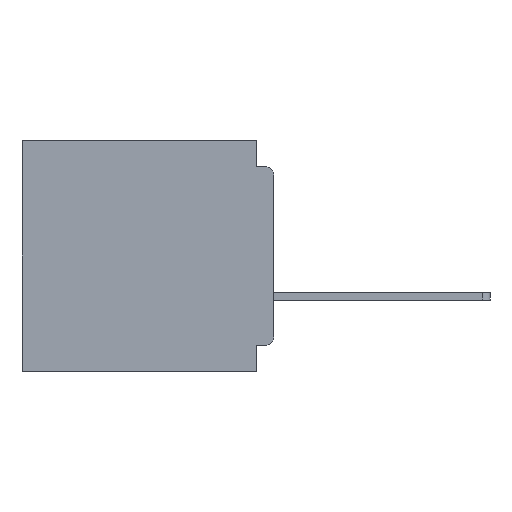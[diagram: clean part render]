
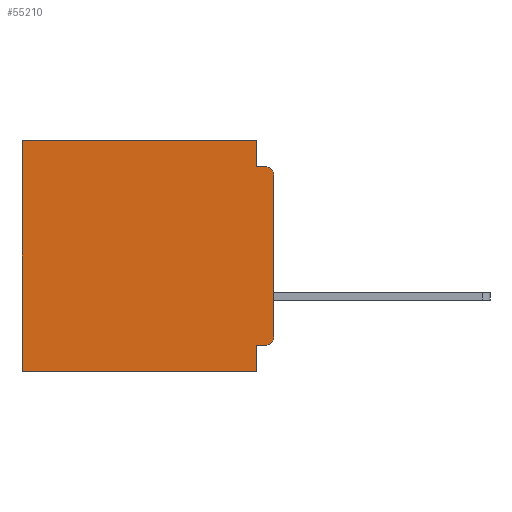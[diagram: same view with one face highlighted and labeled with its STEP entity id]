
A CAD part, left-side view. The second image highlights one B-rep face of the part: STEP entity #55210.
In plain terms, the highlighted planar face has unit normal (-1, 0, 0).
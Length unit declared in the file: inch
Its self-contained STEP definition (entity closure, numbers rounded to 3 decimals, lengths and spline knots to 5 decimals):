
#188 = VERTEX_POINT ( 'NONE', #54614 ) ;
#977 = VECTOR ( 'NONE', #39363, 39.37008 ) ;
#2365 = DIRECTION ( 'NONE',  ( -1., 0., 0. ) ) ;
#2395 = ORIENTED_EDGE ( 'NONE', *, *, #59650, .F. ) ;
#2439 = VERTEX_POINT ( 'NONE', #23832 ) ;
#3123 = CARTESIAN_POINT ( 'NONE',  ( 0.3, 0.031, -0.4 ) ) ;
#3156 = ORIENTED_EDGE ( 'NONE', *, *, #58411, .T. ) ;
#3273 = ORIENTED_EDGE ( 'NONE', *, *, #16764, .T. ) ;
#4020 = ORIENTED_EDGE ( 'NONE', *, *, #51384, .F. ) ;
#4127 = LINE ( 'NONE', #34115, #977 ) ;
#4299 = VERTEX_POINT ( 'NONE', #32899 ) ;
#4780 = DIRECTION ( 'NONE',  ( 0., -1., 0. ) ) ;
#5477 = LINE ( 'NONE', #53303, #43898 ) ;
#5922 = EDGE_LOOP ( 'NONE', ( #36828, #3156, #2395, #48694, #37758, #15868, #4020, #22206, #10386, #3273 ) ) ;
#6091 = VERTEX_POINT ( 'NONE', #54589 ) ;
#6470 = EDGE_CURVE ( 'NONE', #27082, #53759, #19765, .T. ) ;
#8656 = VERTEX_POINT ( 'NONE', #11162 ) ;
#10386 = ORIENTED_EDGE ( 'NONE', *, *, #46397, .F. ) ;
#10710 = DIRECTION ( 'NONE',  ( 0., 1., 0. ) ) ;
#11162 = CARTESIAN_POINT ( 'NONE',  ( 0.3, 0.015, -0.045 ) ) ;
#11356 = DIRECTION ( 'NONE',  ( -1., 0., 0. ) ) ;
#14209 = VERTEX_POINT ( 'NONE', #3123 ) ;
#14548 = CARTESIAN_POINT ( 'NONE',  ( 0.3, 0.031, -0.4 ) ) ;
#15117 = VERTEX_POINT ( 'NONE', #15348 ) ;
#15348 = CARTESIAN_POINT ( 'NONE',  ( 0.3, 0., -0.34 ) ) ;
#15868 = ORIENTED_EDGE ( 'NONE', *, *, #6470, .T. ) ;
#16097 = DIRECTION ( 'NONE',  ( 0., 1., 0. ) ) ;
#16764 = EDGE_CURVE ( 'NONE', #188, #15117, #54181, .T. ) ;
#18435 = DIRECTION ( 'NONE',  ( 1., 0., 0. ) ) ;
#19655 = DIRECTION ( 'NONE',  ( 0., 0., -1. ) ) ;
#19765 = LINE ( 'NONE', #42918, #31471 ) ;
#20411 = EDGE_CURVE ( 'NONE', #2439, #15117, #5477, .T. ) ;
#22071 = VECTOR ( 'NONE', #28201, 39.37008 ) ;
#22206 = ORIENTED_EDGE ( 'NONE', *, *, #30041, .F. ) ;
#23205 = CARTESIAN_POINT ( 'NONE',  ( 0.3, 0., -0.355 ) ) ;
#23832 = CARTESIAN_POINT ( 'NONE',  ( 0.3, 0., -0.06 ) ) ;
#24019 = EDGE_CURVE ( 'NONE', #4299, #6091, #4127, .T. ) ;
#26045 = CARTESIAN_POINT ( 'NONE',  ( 0.3, 0.437, -0.4 ) ) ;
#26183 = CARTESIAN_POINT ( 'NONE',  ( 0.3, 0., 0. ) ) ;
#27082 = VERTEX_POINT ( 'NONE', #36592 ) ;
#28201 = DIRECTION ( 'NONE',  ( 0., 1., 0. ) ) ;
#28497 = CARTESIAN_POINT ( 'NONE',  ( 0.3, 0., -0.4 ) ) ;
#29838 = LINE ( 'NONE', #55800, #53272 ) ;
#30041 = EDGE_CURVE ( 'NONE', #62622, #14209, #51720, .T. ) ;
#31471 = VECTOR ( 'NONE', #57969, 39.37008 ) ;
#32436 = CARTESIAN_POINT ( 'NONE',  ( 0.3, 0.015, -0.06 ) ) ;
#32899 = CARTESIAN_POINT ( 'NONE',  ( 0.3, 0.031, 0. ) ) ;
#33506 = DIRECTION ( 'NONE',  ( 0., 0., -1. ) ) ;
#34115 = CARTESIAN_POINT ( 'NONE',  ( 0.3, 0.031, 0. ) ) ;
#35588 = AXIS2_PLACEMENT_3D ( 'NONE', #32436, #2365, #37455 ) ;
#36509 = FACE_OUTER_BOUND ( 'NONE', #5922, .T. ) ;
#36592 = CARTESIAN_POINT ( 'NONE',  ( 0.3, 0.437, 0. ) ) ;
#36828 = ORIENTED_EDGE ( 'NONE', *, *, #20411, .F. ) ;
#37261 = AXIS2_PLACEMENT_3D ( 'NONE', #41347, #11356, #46363 ) ;
#37455 = DIRECTION ( 'NONE',  ( 0., 0., -1. ) ) ;
#37758 = ORIENTED_EDGE ( 'NONE', *, *, #46779, .T. ) ;
#39363 = DIRECTION ( 'NONE',  ( 0., 0., -1. ) ) ;
#39865 = VECTOR ( 'NONE', #4780, 39.37008 ) ;
#40639 = CARTESIAN_POINT ( 'NONE',  ( 0.3, 0.031, -0.355 ) ) ;
#41347 = CARTESIAN_POINT ( 'NONE',  ( 0.3, 0.015, -0.34 ) ) ;
#41455 = LINE ( 'NONE', #44694, #39865 ) ;
#42918 = CARTESIAN_POINT ( 'NONE',  ( 0.3, 0.437, -0.4 ) ) ;
#43898 = VECTOR ( 'NONE', #48274, 39.37008 ) ;
#44694 = CARTESIAN_POINT ( 'NONE',  ( 0.3, 0., -0.045 ) ) ;
#46363 = DIRECTION ( 'NONE',  ( 0., 0., -1. ) ) ;
#46397 = EDGE_CURVE ( 'NONE', #188, #62622, #48621, .T. ) ;
#46779 = EDGE_CURVE ( 'NONE', #4299, #27082, #64856, .T. ) ;
#48274 = DIRECTION ( 'NONE',  ( 0., 0., -1. ) ) ;
#48621 = LINE ( 'NONE', #23205, #22071 ) ;
#48694 = ORIENTED_EDGE ( 'NONE', *, *, #24019, .F. ) ;
#50153 = VECTOR ( 'NONE', #19655, 39.37008 ) ;
#51384 = EDGE_CURVE ( 'NONE', #14209, #53759, #29838, .T. ) ;
#51701 = VECTOR ( 'NONE', #16097, 39.37008 ) ;
#51720 = LINE ( 'NONE', #14548, #50153 ) ;
#52649 = AXIS2_PLACEMENT_3D ( 'NONE', #28497, #18435, #33506 ) ;
#53272 = VECTOR ( 'NONE', #10710, 39.37008 ) ;
#53303 = CARTESIAN_POINT ( 'NONE',  ( 0.3, 0., -0.4 ) ) ;
#53759 = VERTEX_POINT ( 'NONE', #26045 ) ;
#54181 = CIRCLE ( 'NONE', #37261, 0.015 ) ;
#54589 = CARTESIAN_POINT ( 'NONE',  ( 0.3, 0.031, -0.045 ) ) ;
#54614 = CARTESIAN_POINT ( 'NONE',  ( 0.3, 0.015, -0.355 ) ) ;
#55210 = ADVANCED_FACE ( 'NONE', ( #36509 ), #58393, .F. ) ;
#55800 = CARTESIAN_POINT ( 'NONE',  ( 0.3, 0., -0.4 ) ) ;
#56510 = CIRCLE ( 'NONE', #35588, 0.015 ) ;
#57969 = DIRECTION ( 'NONE',  ( 0., 0., -1. ) ) ;
#58393 = PLANE ( 'NONE',  #52649 ) ;
#58411 = EDGE_CURVE ( 'NONE', #2439, #8656, #56510, .T. ) ;
#59650 = EDGE_CURVE ( 'NONE', #6091, #8656, #41455, .T. ) ;
#62622 = VERTEX_POINT ( 'NONE', #40639 ) ;
#64856 = LINE ( 'NONE', #26183, #51701 ) ;
